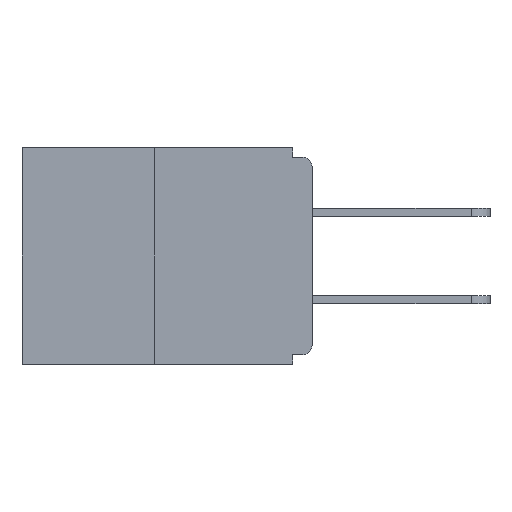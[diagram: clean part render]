
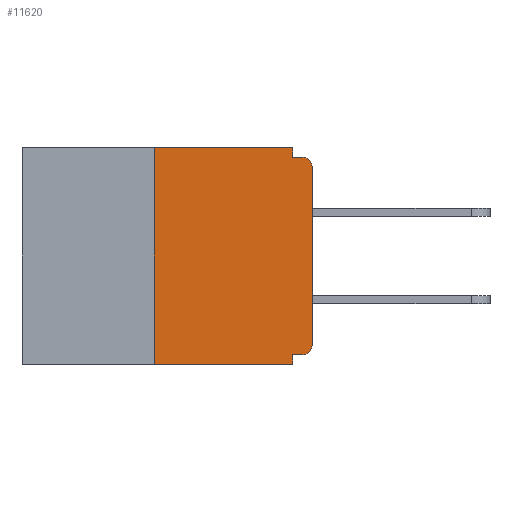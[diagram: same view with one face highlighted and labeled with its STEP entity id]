
A CAD part, left-side view. The second image highlights one B-rep face of the part: STEP entity #11620.
In plain terms, the highlighted planar face has unit normal (-1, 0, 0).
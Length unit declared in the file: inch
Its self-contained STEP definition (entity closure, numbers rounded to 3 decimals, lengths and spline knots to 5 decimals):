
#324 = CARTESIAN_POINT ( 'NONE',  ( 0., 0.031, -0.343 ) ) ;
#361 = VERTEX_POINT ( 'NONE', #12715 ) ;
#747 = ORIENTED_EDGE ( 'NONE', *, *, #11373, .F. ) ;
#1530 = CARTESIAN_POINT ( 'NONE',  ( 0., 0.031, 0. ) ) ;
#1563 = CIRCLE ( 'NONE', #22385, 0.015 ) ;
#1572 = CARTESIAN_POINT ( 'NONE',  ( 0., 0.25, -0.343 ) ) ;
#1601 = CARTESIAN_POINT ( 'NONE',  ( 0., 0.015, -0.03 ) ) ;
#2123 = FACE_OUTER_BOUND ( 'NONE', #20692, .T. ) ;
#2955 = DIRECTION ( 'NONE',  ( -1., 0., 0. ) ) ;
#2978 = DIRECTION ( 'NONE',  ( 0., 0., -1. ) ) ;
#3176 = EDGE_CURVE ( 'NONE', #3632, #361, #4962, .T. ) ;
#3509 = EDGE_CURVE ( 'NONE', #9144, #16034, #21105, .T. ) ;
#3632 = VERTEX_POINT ( 'NONE', #19107 ) ;
#3897 = DIRECTION ( 'NONE',  ( 0., -1., 0. ) ) ;
#3911 = ORIENTED_EDGE ( 'NONE', *, *, #20495, .F. ) ;
#4192 = LINE ( 'NONE', #20128, #8820 ) ;
#4625 = DIRECTION ( 'NONE',  ( 0., 0., -1. ) ) ;
#4857 = LINE ( 'NONE', #18249, #6485 ) ;
#4962 = LINE ( 'NONE', #16101, #6854 ) ;
#5577 = DIRECTION ( 'NONE',  ( 0., 0., -1. ) ) ;
#6459 = CARTESIAN_POINT ( 'NONE',  ( 0., 0.031, 0. ) ) ;
#6462 = ORIENTED_EDGE ( 'NONE', *, *, #15014, .F. ) ;
#6485 = VECTOR ( 'NONE', #7276, 39.37008 ) ;
#6775 = EDGE_CURVE ( 'NONE', #14555, #16958, #4857, .T. ) ;
#6835 = CARTESIAN_POINT ( 'NONE',  ( 0., 0.031, -0.328 ) ) ;
#6854 = VECTOR ( 'NONE', #3897, 39.37008 ) ;
#7276 = DIRECTION ( 'NONE',  ( 0., 0., 1. ) ) ;
#7458 = VECTOR ( 'NONE', #14628, 39.37008 ) ;
#8000 = ORIENTED_EDGE ( 'NONE', *, *, #6775, .F. ) ;
#8216 = ORIENTED_EDGE ( 'NONE', *, *, #12207, .T. ) ;
#8369 = VECTOR ( 'NONE', #11470, 39.37008 ) ;
#8484 = ORIENTED_EDGE ( 'NONE', *, *, #22477, .T. ) ;
#8525 = PLANE ( 'NONE',  #14260 ) ;
#8624 = EDGE_CURVE ( 'NONE', #10773, #3632, #22057, .T. ) ;
#8820 = VECTOR ( 'NONE', #9655, 39.37008 ) ;
#9144 = VERTEX_POINT ( 'NONE', #16533 ) ;
#9371 = ORIENTED_EDGE ( 'NONE', *, *, #3509, .T. ) ;
#9496 = EDGE_CURVE ( 'NONE', #16034, #14137, #9685, .T. ) ;
#9655 = DIRECTION ( 'NONE',  ( 0., -1., 0. ) ) ;
#9685 = LINE ( 'NONE', #10616, #7458 ) ;
#9794 = CARTESIAN_POINT ( 'NONE',  ( 0., 0.46, -0.343 ) ) ;
#10616 = CARTESIAN_POINT ( 'NONE',  ( 0., 0., 0. ) ) ;
#10726 = VERTEX_POINT ( 'NONE', #6835 ) ;
#10773 = VERTEX_POINT ( 'NONE', #1530 ) ;
#11240 = AXIS2_PLACEMENT_3D ( 'NONE', #15311, #2955, #4625 ) ;
#11373 = EDGE_CURVE ( 'NONE', #16958, #10773, #4192, .T. ) ;
#11470 = DIRECTION ( 'NONE',  ( 0., -1., 0. ) ) ;
#11620 = ADVANCED_FACE ( 'NONE', ( #2123 ), #8525, .F. ) ;
#11771 = CARTESIAN_POINT ( 'NONE',  ( 0., 0., -0.03 ) ) ;
#11774 = VECTOR ( 'NONE', #5577, 39.37008 ) ;
#12207 = EDGE_CURVE ( 'NONE', #14137, #361, #1563, .T. ) ;
#12561 = ORIENTED_EDGE ( 'NONE', *, *, #9496, .T. ) ;
#12610 = DIRECTION ( 'NONE',  ( 1., 0., 0. ) ) ;
#12715 = CARTESIAN_POINT ( 'NONE',  ( 0., 0.015, -0.015 ) ) ;
#13471 = VECTOR ( 'NONE', #13478, 39.37008 ) ;
#13478 = DIRECTION ( 'NONE',  ( 0., 1., 0. ) ) ;
#14137 = VERTEX_POINT ( 'NONE', #11771 ) ;
#14260 = AXIS2_PLACEMENT_3D ( 'NONE', #15551, #12610, #21072 ) ;
#14555 = VERTEX_POINT ( 'NONE', #1572 ) ;
#14628 = DIRECTION ( 'NONE',  ( 0., 0., 1. ) ) ;
#15014 = EDGE_CURVE ( 'NONE', #9144, #10726, #20882, .T. ) ;
#15311 = CARTESIAN_POINT ( 'NONE',  ( 0., 0.015, -0.313 ) ) ;
#15551 = CARTESIAN_POINT ( 'NONE',  ( 0., 0.46, 0. ) ) ;
#16034 = VERTEX_POINT ( 'NONE', #21420 ) ;
#16101 = CARTESIAN_POINT ( 'NONE',  ( 0., 0., -0.015 ) ) ;
#16533 = CARTESIAN_POINT ( 'NONE',  ( 0., 0.015, -0.328 ) ) ;
#16958 = VERTEX_POINT ( 'NONE', #18791 ) ;
#17059 = CARTESIAN_POINT ( 'NONE',  ( 0., 0., -0.328 ) ) ;
#17574 = VERTEX_POINT ( 'NONE', #18805 ) ;
#17624 = VECTOR ( 'NONE', #2978, 39.37008 ) ;
#17634 = LINE ( 'NONE', #9794, #8369 ) ;
#18249 = CARTESIAN_POINT ( 'NONE',  ( 0., 0.25, 0. ) ) ;
#18791 = CARTESIAN_POINT ( 'NONE',  ( 0., 0.25, 0. ) ) ;
#18805 = CARTESIAN_POINT ( 'NONE',  ( 0., 0.031, -0.343 ) ) ;
#19107 = CARTESIAN_POINT ( 'NONE',  ( 0., 0.031, -0.015 ) ) ;
#19280 = ORIENTED_EDGE ( 'NONE', *, *, #3176, .F. ) ;
#19719 = DIRECTION ( 'NONE',  ( -1., 0., 0. ) ) ;
#20128 = CARTESIAN_POINT ( 'NONE',  ( 0., 0.46, 0. ) ) ;
#20495 = EDGE_CURVE ( 'NONE', #10726, #17574, #21882, .T. ) ;
#20692 = EDGE_LOOP ( 'NONE', ( #747, #8000, #8484, #3911, #6462, #9371, #12561, #8216, #19280, #21611 ) ) ;
#20882 = LINE ( 'NONE', #17059, #13471 ) ;
#21072 = DIRECTION ( 'NONE',  ( 0., 0., -1. ) ) ;
#21105 = CIRCLE ( 'NONE', #11240, 0.015 ) ;
#21420 = CARTESIAN_POINT ( 'NONE',  ( 0., 0., -0.313 ) ) ;
#21515 = DIRECTION ( 'NONE',  ( 0., 0., -1. ) ) ;
#21611 = ORIENTED_EDGE ( 'NONE', *, *, #8624, .F. ) ;
#21882 = LINE ( 'NONE', #324, #11774 ) ;
#22057 = LINE ( 'NONE', #6459, #17624 ) ;
#22385 = AXIS2_PLACEMENT_3D ( 'NONE', #1601, #19719, #21515 ) ;
#22477 = EDGE_CURVE ( 'NONE', #14555, #17574, #17634, .T. ) ;
